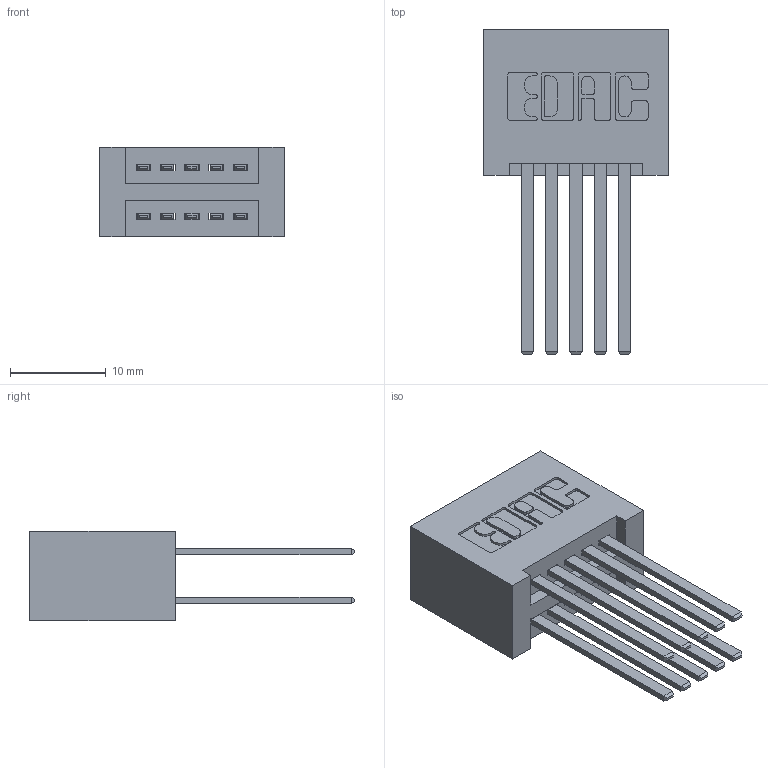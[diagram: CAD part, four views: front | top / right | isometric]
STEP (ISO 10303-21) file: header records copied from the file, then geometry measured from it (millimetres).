
FILE_DESCRIPTION (( 'STEP AP203' ), '1' );
FILE_NAME ('345-010-544-201.STEP', '2019-10-26T14:27:53', ( '' ), ( '' ), 'SwSTEP 2.0', 'SolidWorks 2016', '' );
FILE_SCHEMA (( 'CONFIG_CONTROL_DESIGN' ));
Length unit declared in the file: inch
Products named in the file (3): 345-010-544-201; 345 Part_No Mounting Lugs; 345-292-001_345-293-144
Assembly tree (11 placements, depth 2):
  345-010-544-201
    345 Part_No Mounting Lugs
    345-292-001_345-293-144  x10
Bounding box: 19.3 x 33.96 x 9.4 mm (x, y, z)
Volume: 2287.9 mm3; surface area: 3379.3 mm2
Topology: 11 solids, 11 shells, 558 faces, 1627 edges, 1070 vertices
Faces by surface type: plane 366, cylinder 192
Entity records: 8443 total; most frequent: CARTESIAN_POINT 1448, ORIENTED_EDGE 1382, DIRECTION 1315, EDGE_CURVE 691, VECTOR 551, LINE 551, VERTEX_POINT 458, AXIS2_PLACEMENT_3D 382
